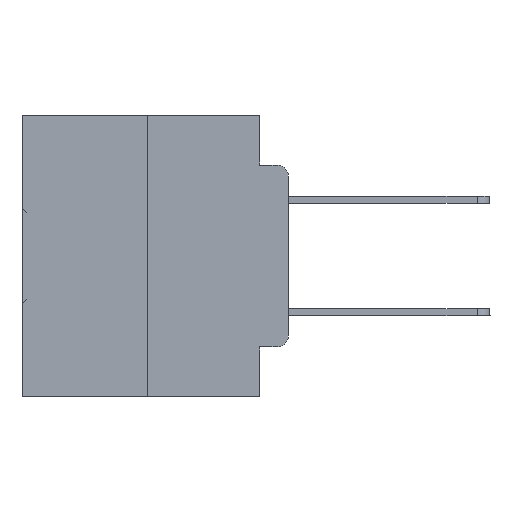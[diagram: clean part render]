
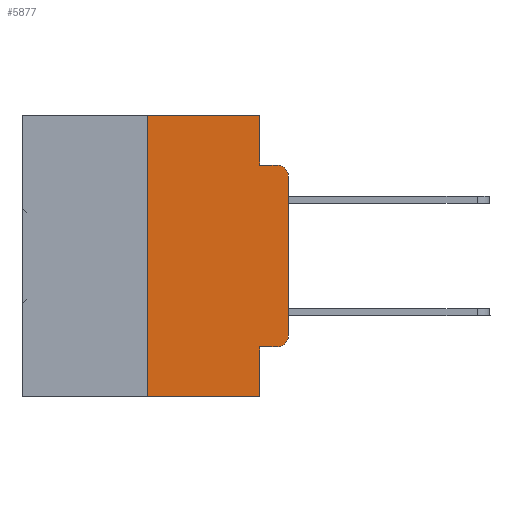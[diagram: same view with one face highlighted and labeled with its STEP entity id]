
A CAD part, left-side view. The second image highlights one B-rep face of the part: STEP entity #5877.
In plain terms, the highlighted planar face has unit normal (-1, 0, 0).
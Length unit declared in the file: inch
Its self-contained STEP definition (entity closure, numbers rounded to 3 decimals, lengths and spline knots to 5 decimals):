
#3 = VERTEX_POINT ( 'NONE', #3759 ) ;
#741 = ORIENTED_EDGE ( 'NONE', *, *, #5833, .T. ) ;
#784 = CARTESIAN_POINT ( 'NONE',  ( 0., 0.051, -0.0885 ) ) ;
#945 = EDGE_CURVE ( 'NONE', #8186, #34275, #3175, .T. ) ;
#2303 = DIRECTION ( 'NONE',  ( 0., 0., -1. ) ) ;
#3126 = EDGE_CURVE ( 'NONE', #8186, #17792, #11902, .T. ) ;
#3175 = LINE ( 'NONE', #29608, #30732 ) ;
#3533 = AXIS2_PLACEMENT_3D ( 'NONE', #34830, #24180, #15972 ) ;
#3759 = CARTESIAN_POINT ( 'NONE',  ( 0., 0., -0.3915 ) ) ;
#4011 = CARTESIAN_POINT ( 'NONE',  ( 0., 0.473, 0. ) ) ;
#4138 = CARTESIAN_POINT ( 'NONE',  ( 0., 0.051, -0.4115 ) ) ;
#4249 = VECTOR ( 'NONE', #29238, 39.37008 ) ;
#4843 = ORIENTED_EDGE ( 'NONE', *, *, #18055, .T. ) ;
#5248 = CARTESIAN_POINT ( 'NONE',  ( 0., 0.25, 0. ) ) ;
#5369 = VECTOR ( 'NONE', #2303, 39.37008 ) ;
#5738 = CARTESIAN_POINT ( 'NONE',  ( 0., 0.051, -0.5 ) ) ;
#5833 = EDGE_CURVE ( 'NONE', #31698, #21035, #8676, .T. ) ;
#5877 = ADVANCED_FACE ( 'NONE', ( #25191 ), #14746, .F. ) ;
#5887 = ORIENTED_EDGE ( 'NONE', *, *, #32406, .F. ) ;
#7188 = CIRCLE ( 'NONE', #3533, 0.02 ) ;
#7334 = EDGE_CURVE ( 'NONE', #21035, #3, #28095, .T. ) ;
#8186 = VERTEX_POINT ( 'NONE', #19557 ) ;
#8676 = LINE ( 'NONE', #4138, #32031 ) ;
#9308 = DIRECTION ( 'NONE',  ( 0., -1., 0. ) ) ;
#11313 = VERTEX_POINT ( 'NONE', #28805 ) ;
#11320 = AXIS2_PLACEMENT_3D ( 'NONE', #19595, #22338, #17103 ) ;
#11818 = EDGE_CURVE ( 'NONE', #34275, #23232, #22276, .T. ) ;
#11902 = LINE ( 'NONE', #18121, #19948 ) ;
#12146 = CARTESIAN_POINT ( 'NONE',  ( 0., 0.02, -0.4115 ) ) ;
#12215 = EDGE_CURVE ( 'NONE', #34388, #11313, #7188, .T. ) ;
#13211 = CARTESIAN_POINT ( 'NONE',  ( 0., 0.051, 0. ) ) ;
#14746 = PLANE ( 'NONE',  #15382 ) ;
#15382 = AXIS2_PLACEMENT_3D ( 'NONE', #4011, #22940, #31475 ) ;
#15443 = ORIENTED_EDGE ( 'NONE', *, *, #11818, .F. ) ;
#15547 = EDGE_CURVE ( 'NONE', #31698, #17792, #16876, .T. ) ;
#15972 = DIRECTION ( 'NONE',  ( 0., 0., -1. ) ) ;
#16544 = LINE ( 'NONE', #30376, #20825 ) ;
#16876 = LINE ( 'NONE', #13211, #4249 ) ;
#17103 = DIRECTION ( 'NONE',  ( 0., 0., -1. ) ) ;
#17423 = CARTESIAN_POINT ( 'NONE',  ( 0., 0.051, 0. ) ) ;
#17475 = CARTESIAN_POINT ( 'NONE',  ( 0., 0.473, 0. ) ) ;
#17698 = DIRECTION ( 'NONE',  ( 0., 0., 1. ) ) ;
#17792 = VERTEX_POINT ( 'NONE', #5738 ) ;
#18055 = EDGE_CURVE ( 'NONE', #3, #34388, #31637, .T. ) ;
#18121 = CARTESIAN_POINT ( 'NONE',  ( 0., 0.473, -0.5 ) ) ;
#18219 = DIRECTION ( 'NONE',  ( 0., -1., 0. ) ) ;
#19146 = DIRECTION ( 'NONE',  ( 0., -1., 0. ) ) ;
#19557 = CARTESIAN_POINT ( 'NONE',  ( 0., 0.25, -0.5 ) ) ;
#19595 = CARTESIAN_POINT ( 'NONE',  ( 0., 0.02, -0.3915 ) ) ;
#19688 = EDGE_CURVE ( 'NONE', #23232, #33396, #26971, .T. ) ;
#19765 = ORIENTED_EDGE ( 'NONE', *, *, #7334, .T. ) ;
#19948 = VECTOR ( 'NONE', #18219, 39.37008 ) ;
#20825 = VECTOR ( 'NONE', #19146, 39.37008 ) ;
#21035 = VERTEX_POINT ( 'NONE', #12146 ) ;
#22276 = LINE ( 'NONE', #17475, #28694 ) ;
#22338 = DIRECTION ( 'NONE',  ( -1., 0., 0. ) ) ;
#22692 = ORIENTED_EDGE ( 'NONE', *, *, #15547, .F. ) ;
#22705 = VECTOR ( 'NONE', #17698, 39.37008 ) ;
#22940 = DIRECTION ( 'NONE',  ( 1., 0., 0. ) ) ;
#23232 = VERTEX_POINT ( 'NONE', #17423 ) ;
#23411 = CARTESIAN_POINT ( 'NONE',  ( 0., 0., 0. ) ) ;
#24180 = DIRECTION ( 'NONE',  ( -1., 0., 0. ) ) ;
#24698 = ORIENTED_EDGE ( 'NONE', *, *, #12215, .T. ) ;
#25191 = FACE_OUTER_BOUND ( 'NONE', #30475, .T. ) ;
#26971 = LINE ( 'NONE', #34504, #5369 ) ;
#27219 = ORIENTED_EDGE ( 'NONE', *, *, #945, .F. ) ;
#28095 = CIRCLE ( 'NONE', #11320, 0.02 ) ;
#28694 = VECTOR ( 'NONE', #31374, 39.37008 ) ;
#28805 = CARTESIAN_POINT ( 'NONE',  ( 0., 0.02, -0.0885 ) ) ;
#29238 = DIRECTION ( 'NONE',  ( 0., 0., -1. ) ) ;
#29608 = CARTESIAN_POINT ( 'NONE',  ( 0., 0.25, 0. ) ) ;
#29995 = CARTESIAN_POINT ( 'NONE',  ( 0., 0.051, -0.4115 ) ) ;
#30376 = CARTESIAN_POINT ( 'NONE',  ( 0., 0.051, -0.0885 ) ) ;
#30475 = EDGE_LOOP ( 'NONE', ( #4843, #24698, #5887, #34628, #15443, #27219, #33581, #22692, #741, #19765 ) ) ;
#30732 = VECTOR ( 'NONE', #34905, 39.37008 ) ;
#31374 = DIRECTION ( 'NONE',  ( 0., -1., 0. ) ) ;
#31475 = DIRECTION ( 'NONE',  ( 0., 0., -1. ) ) ;
#31637 = LINE ( 'NONE', #23411, #22705 ) ;
#31698 = VERTEX_POINT ( 'NONE', #29995 ) ;
#32031 = VECTOR ( 'NONE', #9308, 39.37008 ) ;
#32406 = EDGE_CURVE ( 'NONE', #33396, #11313, #16544, .T. ) ;
#32537 = CARTESIAN_POINT ( 'NONE',  ( 0., 0., -0.1085 ) ) ;
#33396 = VERTEX_POINT ( 'NONE', #784 ) ;
#33581 = ORIENTED_EDGE ( 'NONE', *, *, #3126, .T. ) ;
#34275 = VERTEX_POINT ( 'NONE', #5248 ) ;
#34388 = VERTEX_POINT ( 'NONE', #32537 ) ;
#34504 = CARTESIAN_POINT ( 'NONE',  ( 0., 0.051, 0. ) ) ;
#34628 = ORIENTED_EDGE ( 'NONE', *, *, #19688, .F. ) ;
#34830 = CARTESIAN_POINT ( 'NONE',  ( 0., 0.02, -0.1085 ) ) ;
#34905 = DIRECTION ( 'NONE',  ( 0., 0., 1. ) ) ;
